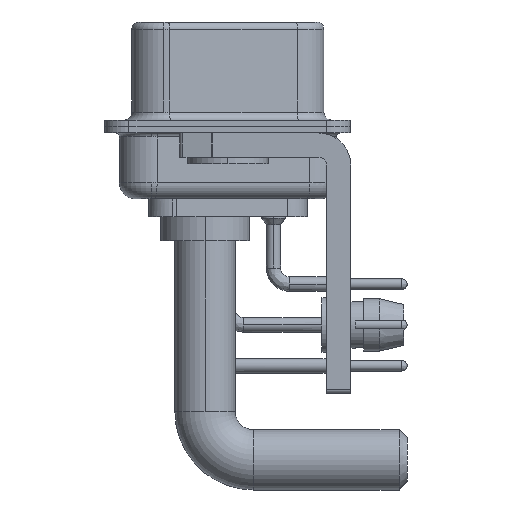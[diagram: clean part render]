
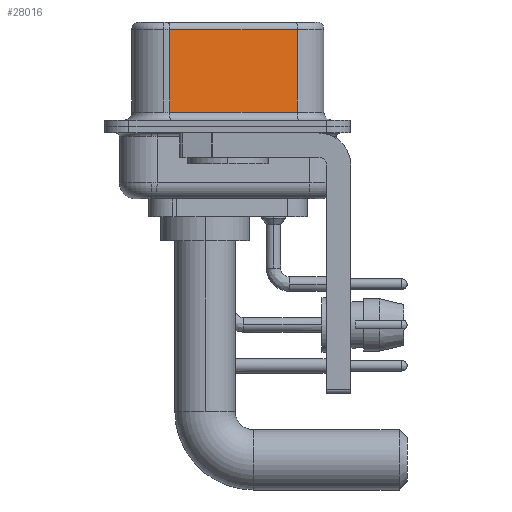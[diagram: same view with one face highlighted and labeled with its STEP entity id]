
A CAD part, left-side view. The second image highlights one B-rep face of the part: STEP entity #28016.
In plain terms, the highlighted planar face has unit normal (-0.985, -0.174, 0).
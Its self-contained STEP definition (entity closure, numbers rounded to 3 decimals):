
#156 = VERTEX_POINT ( 'NONE', #10922 ) ;
#1158 = CARTESIAN_POINT ( 'NONE',  ( 5.132, -4.322, 0.9 ) ) ;
#1331 = LINE ( 'NONE', #10421, #32294 ) ;
#3769 = CARTESIAN_POINT ( 'NONE',  ( 5.132, -4.322, 6.02 ) ) ;
#4128 = DIRECTION ( 'NONE',  ( -0.174, 0.985, 0. ) ) ;
#6133 = VERTEX_POINT ( 'NONE', #8400 ) ;
#6731 = LINE ( 'NONE', #3769, #31088 ) ;
#8400 = CARTESIAN_POINT ( 'NONE',  ( 5.132, -4.322, 0.9 ) ) ;
#9525 = LINE ( 'NONE', #1158, #16547 ) ;
#9889 = DIRECTION ( 'NONE',  ( 0.174, -0.985, 0. ) ) ;
#10421 = CARTESIAN_POINT ( 'NONE',  ( 3.73, 3.628, 6.52 ) ) ;
#10573 = CARTESIAN_POINT ( 'NONE',  ( 5.132, -4.322, 6.02 ) ) ;
#10922 = CARTESIAN_POINT ( 'NONE',  ( 3.73, 3.628, 0.9 ) ) ;
#11266 = EDGE_CURVE ( 'NONE', #28030, #6133, #26330, .T. ) ;
#12287 = EDGE_CURVE ( 'NONE', #20913, #156, #1331, .T. ) ;
#15950 = CARTESIAN_POINT ( 'NONE',  ( 5.132, -4.322, 6.52 ) ) ;
#16477 = ORIENTED_EDGE ( 'NONE', *, *, #27294, .T. ) ;
#16547 = VECTOR ( 'NONE', #9889, 1000. ) ;
#17095 = ORIENTED_EDGE ( 'NONE', *, *, #12287, .T. ) ;
#17308 = EDGE_CURVE ( 'NONE', #156, #6133, #9525, .T. ) ;
#17827 = ORIENTED_EDGE ( 'NONE', *, *, #17308, .T. ) ;
#17964 = ORIENTED_EDGE ( 'NONE', *, *, #11266, .F. ) ;
#20053 = CARTESIAN_POINT ( 'NONE',  ( 5.132, -4.322, 6.52 ) ) ;
#20807 = EDGE_LOOP ( 'NONE', ( #17964, #16477, #17095, #17827 ) ) ;
#20913 = VERTEX_POINT ( 'NONE', #29396 ) ;
#21507 = PLANE ( 'NONE',  #22308 ) ;
#21722 = DIRECTION ( 'NONE',  ( 0., 0., -1. ) ) ;
#22308 = AXIS2_PLACEMENT_3D ( 'NONE', #15950, #27244, #24472 ) ;
#24472 = DIRECTION ( 'NONE',  ( -0.174, 0.985, 0. ) ) ;
#26330 = LINE ( 'NONE', #20053, #32297 ) ;
#27244 = DIRECTION ( 'NONE',  ( 0.985, 0.174, 0. ) ) ;
#27294 = EDGE_CURVE ( 'NONE', #28030, #20913, #6731, .T. ) ;
#28016 = ADVANCED_FACE ( 'NONE', ( #30556 ), #21507, .F. ) ;
#28030 = VERTEX_POINT ( 'NONE', #10573 ) ;
#29396 = CARTESIAN_POINT ( 'NONE',  ( 3.73, 3.628, 6.02 ) ) ;
#30556 = FACE_OUTER_BOUND ( 'NONE', #20807, .T. ) ;
#31088 = VECTOR ( 'NONE', #4128, 1000. ) ;
#31486 = DIRECTION ( 'NONE',  ( 0., 0., -1. ) ) ;
#32294 = VECTOR ( 'NONE', #21722, 1000. ) ;
#32297 = VECTOR ( 'NONE', #31486, 1000. ) ;
